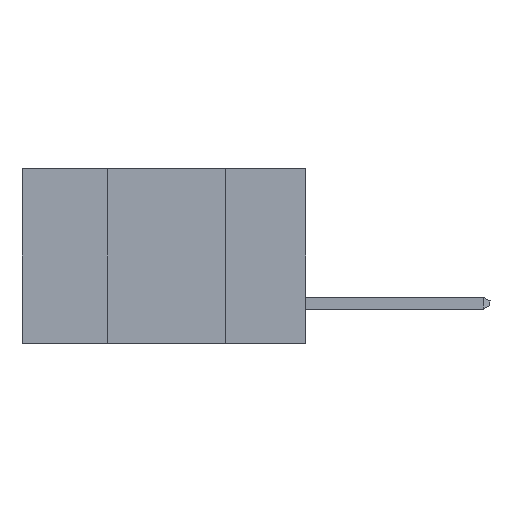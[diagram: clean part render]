
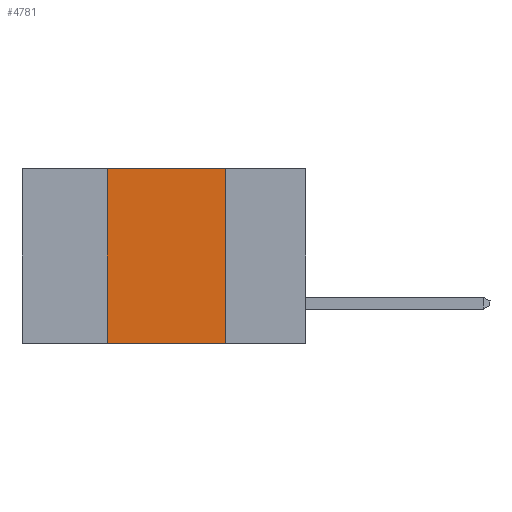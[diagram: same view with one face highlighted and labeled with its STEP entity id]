
A CAD part, left-side view. The second image highlights one B-rep face of the part: STEP entity #4781.
In plain terms, the highlighted planar face has unit normal (-1, 0, 0).
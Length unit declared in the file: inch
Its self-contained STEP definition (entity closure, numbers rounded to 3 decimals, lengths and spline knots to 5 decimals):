
#165 = VERTEX_POINT ( 'NONE', #14871 ) ;
#2111 = VECTOR ( 'NONE', #11933, 39.37008 ) ;
#3535 = LINE ( 'NONE', #19615, #2111 ) ;
#3951 = DIRECTION ( 'NONE',  ( 0., 0., -1. ) ) ;
#4029 = CARTESIAN_POINT ( 'NONE',  ( 0., 0.17, -0.37 ) ) ;
#4591 = VECTOR ( 'NONE', #7977, 39.37008 ) ;
#4781 = ADVANCED_FACE ( 'NONE', ( #22010 ), #24365, .F. ) ;
#5801 = CARTESIAN_POINT ( 'NONE',  ( 0., 0.6, 0. ) ) ;
#6328 = EDGE_LOOP ( 'NONE', ( #22150, #11934, #8457, #9270 ) ) ;
#7234 = VECTOR ( 'NONE', #11300, 39.37008 ) ;
#7977 = DIRECTION ( 'NONE',  ( 0., -1., 0. ) ) ;
#8178 = CARTESIAN_POINT ( 'NONE',  ( 0., 0.42, -0.37 ) ) ;
#8457 = ORIENTED_EDGE ( 'NONE', *, *, #14468, .F. ) ;
#9270 = ORIENTED_EDGE ( 'NONE', *, *, #12798, .T. ) ;
#9982 = VECTOR ( 'NONE', #13540, 39.37008 ) ;
#10768 = VERTEX_POINT ( 'NONE', #8178 ) ;
#11300 = DIRECTION ( 'NONE',  ( 0., 0., 1. ) ) ;
#11920 = CARTESIAN_POINT ( 'NONE',  ( 0., 0.42, 0. ) ) ;
#11933 = DIRECTION ( 'NONE',  ( 0., -1., 0. ) ) ;
#11934 = ORIENTED_EDGE ( 'NONE', *, *, #12036, .F. ) ;
#12036 = EDGE_CURVE ( 'NONE', #16537, #14654, #13519, .T. ) ;
#12798 = EDGE_CURVE ( 'NONE', #10768, #165, #3535, .T. ) ;
#13519 = LINE ( 'NONE', #21946, #4591 ) ;
#13540 = DIRECTION ( 'NONE',  ( 0., 0., -1. ) ) ;
#14354 = DIRECTION ( 'NONE',  ( 1., 0., 0. ) ) ;
#14468 = EDGE_CURVE ( 'NONE', #10768, #16537, #19370, .T. ) ;
#14654 = VERTEX_POINT ( 'NONE', #25697 ) ;
#14871 = CARTESIAN_POINT ( 'NONE',  ( 0., 0.17, -0.37 ) ) ;
#16537 = VERTEX_POINT ( 'NONE', #11920 ) ;
#18737 = AXIS2_PLACEMENT_3D ( 'NONE', #5801, #14354, #3951 ) ;
#19370 = LINE ( 'NONE', #25299, #7234 ) ;
#19478 = LINE ( 'NONE', #4029, #9982 ) ;
#19615 = CARTESIAN_POINT ( 'NONE',  ( 0., 0.6, -0.37 ) ) ;
#21946 = CARTESIAN_POINT ( 'NONE',  ( 0., 0.6, 0. ) ) ;
#22010 = FACE_OUTER_BOUND ( 'NONE', #6328, .T. ) ;
#22150 = ORIENTED_EDGE ( 'NONE', *, *, #23602, .F. ) ;
#23602 = EDGE_CURVE ( 'NONE', #14654, #165, #19478, .T. ) ;
#24365 = PLANE ( 'NONE',  #18737 ) ;
#25299 = CARTESIAN_POINT ( 'NONE',  ( 0., 0.42, -0.37 ) ) ;
#25697 = CARTESIAN_POINT ( 'NONE',  ( 0., 0.17, 0. ) ) ;
